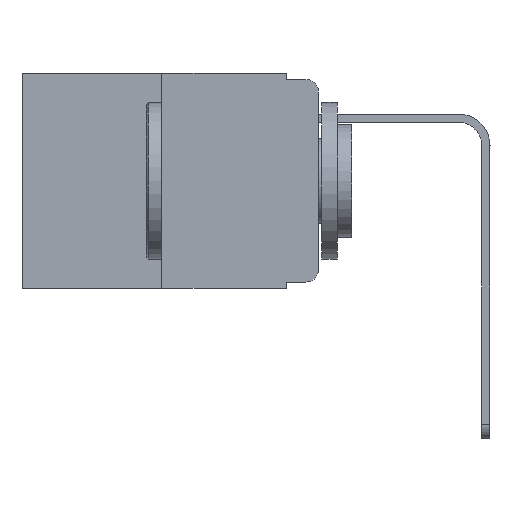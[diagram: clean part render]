
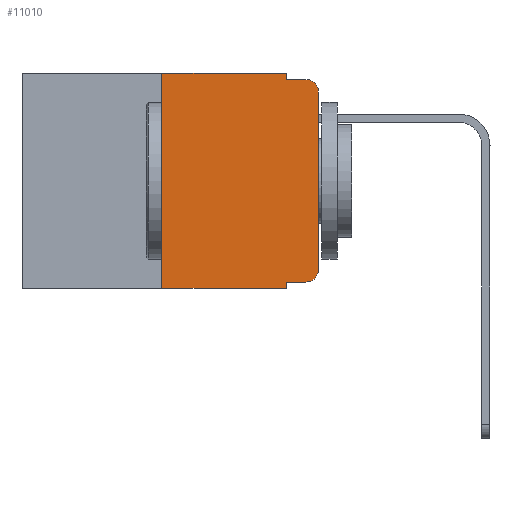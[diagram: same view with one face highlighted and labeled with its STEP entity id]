
A CAD part, left-side view. The second image highlights one B-rep face of the part: STEP entity #11010.
In plain terms, the highlighted planar face has unit normal (-1, 0, 0).
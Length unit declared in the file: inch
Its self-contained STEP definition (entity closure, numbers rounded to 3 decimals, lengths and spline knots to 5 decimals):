
#340 = ORIENTED_EDGE ( 'NONE', *, *, #976, .F. ) ;
#483 = FACE_OUTER_BOUND ( 'NONE', #11737, .T. ) ;
#563 = DIRECTION ( 'NONE',  ( 0., -1., 0. ) ) ;
#676 = ORIENTED_EDGE ( 'NONE', *, *, #8915, .F. ) ;
#771 = VECTOR ( 'NONE', #4059, 39.37008 ) ;
#906 = VECTOR ( 'NONE', #3947, 39.37008 ) ;
#976 = EDGE_CURVE ( 'NONE', #1790, #8829, #11258, .T. ) ;
#1168 = EDGE_CURVE ( 'NONE', #5914, #4375, #9947, .T. ) ;
#1240 = DIRECTION ( 'NONE',  ( 0., 0., -1. ) ) ;
#1279 = DIRECTION ( 'NONE',  ( -1., 0., 0. ) ) ;
#1292 = CARTESIAN_POINT ( 'NONE',  ( 0., 0.051, -0.343 ) ) ;
#1371 = ORIENTED_EDGE ( 'NONE', *, *, #5702, .T. ) ;
#1675 = ORIENTED_EDGE ( 'NONE', *, *, #7313, .T. ) ;
#1790 = VERTEX_POINT ( 'NONE', #2151 ) ;
#1953 = CARTESIAN_POINT ( 'NONE',  ( 0., 0.25, 0. ) ) ;
#2112 = DIRECTION ( 'NONE',  ( 0., 0., -1. ) ) ;
#2140 = CARTESIAN_POINT ( 'NONE',  ( 0., 0., -0.03 ) ) ;
#2151 = CARTESIAN_POINT ( 'NONE',  ( 0., 0.051, 0. ) ) ;
#2155 = ORIENTED_EDGE ( 'NONE', *, *, #1168, .F. ) ;
#2215 = CARTESIAN_POINT ( 'NONE',  ( 0., 0.051, -0.01 ) ) ;
#2450 = AXIS2_PLACEMENT_3D ( 'NONE', #10338, #7611, #12138 ) ;
#2560 = VECTOR ( 'NONE', #1240, 39.37008 ) ;
#2982 = EDGE_CURVE ( 'NONE', #5914, #5256, #3390, .T. ) ;
#3034 = ORIENTED_EDGE ( 'NONE', *, *, #11056, .F. ) ;
#3320 = VERTEX_POINT ( 'NONE', #11850 ) ;
#3363 = CARTESIAN_POINT ( 'NONE',  ( 0., 0.473, -0.343 ) ) ;
#3390 = LINE ( 'NONE', #3363, #9025 ) ;
#3684 = VECTOR ( 'NONE', #7143, 39.37008 ) ;
#3838 = VECTOR ( 'NONE', #7362, 39.37008 ) ;
#3947 = DIRECTION ( 'NONE',  ( 0., 0., 1. ) ) ;
#3961 = AXIS2_PLACEMENT_3D ( 'NONE', #11836, #6139, #6174 ) ;
#4059 = DIRECTION ( 'NONE',  ( 0., 0., -1. ) ) ;
#4095 = VERTEX_POINT ( 'NONE', #5556 ) ;
#4139 = CARTESIAN_POINT ( 'NONE',  ( 0., 0.02, -0.313 ) ) ;
#4276 = LINE ( 'NONE', #4299, #3684 ) ;
#4299 = CARTESIAN_POINT ( 'NONE',  ( 0., 0.473, 0. ) ) ;
#4375 = VERTEX_POINT ( 'NONE', #1953 ) ;
#4398 = DIRECTION ( 'NONE',  ( 0., -1., 0. ) ) ;
#4498 = CARTESIAN_POINT ( 'NONE',  ( 0., 0.02, -0.333 ) ) ;
#4613 = CIRCLE ( 'NONE', #2450, 0.02 ) ;
#4754 = VERTEX_POINT ( 'NONE', #2140 ) ;
#5256 = VERTEX_POINT ( 'NONE', #1292 ) ;
#5355 = VERTEX_POINT ( 'NONE', #11053 ) ;
#5369 = LINE ( 'NONE', #11608, #2560 ) ;
#5556 = CARTESIAN_POINT ( 'NONE',  ( 0., 0.051, -0.333 ) ) ;
#5634 = ORIENTED_EDGE ( 'NONE', *, *, #2982, .T. ) ;
#5702 = EDGE_CURVE ( 'NONE', #7951, #3320, #6214, .T. ) ;
#5807 = ORIENTED_EDGE ( 'NONE', *, *, #7021, .F. ) ;
#5914 = VERTEX_POINT ( 'NONE', #12018 ) ;
#5981 = EDGE_CURVE ( 'NONE', #3320, #4754, #9632, .T. ) ;
#6139 = DIRECTION ( 'NONE',  ( 1., 0., 0. ) ) ;
#6174 = DIRECTION ( 'NONE',  ( 0., 0., -1. ) ) ;
#6214 = CIRCLE ( 'NONE', #10278, 0.02 ) ;
#6997 = ORIENTED_EDGE ( 'NONE', *, *, #5981, .T. ) ;
#7021 = EDGE_CURVE ( 'NONE', #4375, #1790, #4276, .T. ) ;
#7143 = DIRECTION ( 'NONE',  ( 0., -1., 0. ) ) ;
#7194 = CARTESIAN_POINT ( 'NONE',  ( 0., 0., 0. ) ) ;
#7313 = EDGE_CURVE ( 'NONE', #4095, #7951, #9330, .T. ) ;
#7362 = DIRECTION ( 'NONE',  ( 0., 0., 1. ) ) ;
#7388 = DIRECTION ( 'NONE',  ( 0., -1., 0. ) ) ;
#7611 = DIRECTION ( 'NONE',  ( -1., 0., 0. ) ) ;
#7951 = VERTEX_POINT ( 'NONE', #4498 ) ;
#8045 = CARTESIAN_POINT ( 'NONE',  ( 0., 0.051, -0.01 ) ) ;
#8351 = CARTESIAN_POINT ( 'NONE',  ( 0., 0.051, -0.333 ) ) ;
#8573 = ORIENTED_EDGE ( 'NONE', *, *, #10565, .T. ) ;
#8605 = CARTESIAN_POINT ( 'NONE',  ( 0., 0.25, 0. ) ) ;
#8829 = VERTEX_POINT ( 'NONE', #2215 ) ;
#8915 = EDGE_CURVE ( 'NONE', #4095, #5256, #5369, .T. ) ;
#9025 = VECTOR ( 'NONE', #4398, 39.37008 ) ;
#9330 = LINE ( 'NONE', #8351, #11937 ) ;
#9632 = LINE ( 'NONE', #7194, #3838 ) ;
#9658 = CARTESIAN_POINT ( 'NONE',  ( 0., 0.051, 0. ) ) ;
#9947 = LINE ( 'NONE', #8605, #906 ) ;
#9961 = VECTOR ( 'NONE', #563, 39.37008 ) ;
#10278 = AXIS2_PLACEMENT_3D ( 'NONE', #4139, #1279, #2112 ) ;
#10338 = CARTESIAN_POINT ( 'NONE',  ( 0., 0.02, -0.03 ) ) ;
#10565 = EDGE_CURVE ( 'NONE', #4754, #5355, #4613, .T. ) ;
#11010 = ADVANCED_FACE ( 'NONE', ( #483 ), #11058, .F. ) ;
#11053 = CARTESIAN_POINT ( 'NONE',  ( 0., 0.02, -0.01 ) ) ;
#11056 = EDGE_CURVE ( 'NONE', #8829, #5355, #12010, .T. ) ;
#11058 = PLANE ( 'NONE',  #3961 ) ;
#11258 = LINE ( 'NONE', #9658, #771 ) ;
#11608 = CARTESIAN_POINT ( 'NONE',  ( 0., 0.051, 0. ) ) ;
#11737 = EDGE_LOOP ( 'NONE', ( #6997, #8573, #3034, #340, #5807, #2155, #5634, #676, #1675, #1371 ) ) ;
#11836 = CARTESIAN_POINT ( 'NONE',  ( 0., 0.473, 0. ) ) ;
#11850 = CARTESIAN_POINT ( 'NONE',  ( 0., 0., -0.313 ) ) ;
#11937 = VECTOR ( 'NONE', #7388, 39.37008 ) ;
#12010 = LINE ( 'NONE', #8045, #9961 ) ;
#12018 = CARTESIAN_POINT ( 'NONE',  ( 0., 0.25, -0.343 ) ) ;
#12138 = DIRECTION ( 'NONE',  ( 0., 0., -1. ) ) ;
